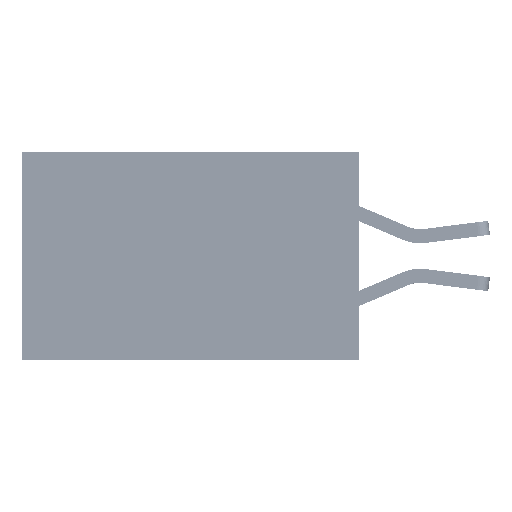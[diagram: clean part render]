
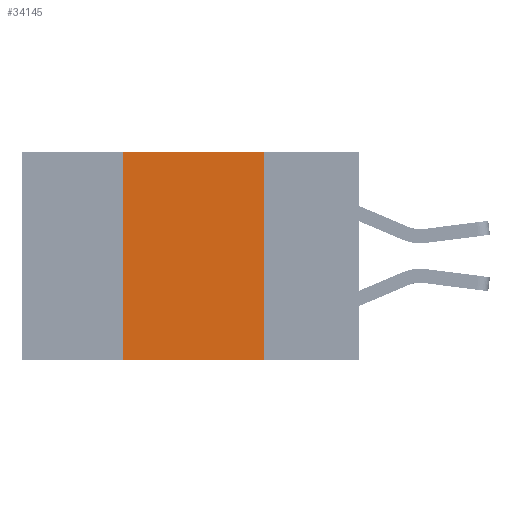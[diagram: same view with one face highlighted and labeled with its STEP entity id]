
A CAD part, left-side view. The second image highlights one B-rep face of the part: STEP entity #34145.
In plain terms, the highlighted planar face has unit normal (-1, 0, 0).
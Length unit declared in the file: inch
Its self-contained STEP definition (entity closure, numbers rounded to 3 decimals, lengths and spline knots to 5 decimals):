
#347 = VECTOR ( 'NONE', #7726, 39.37008 ) ;
#1479 = EDGE_CURVE ( 'NONE', #6688, #5592, #26765, .T. ) ;
#2944 = ORIENTED_EDGE ( 'NONE', *, *, #46217, .F. ) ;
#4751 = ORIENTED_EDGE ( 'NONE', *, *, #13920, .T. ) ;
#5285 = LINE ( 'NONE', #10228, #30888 ) ;
#5592 = VERTEX_POINT ( 'NONE', #26755 ) ;
#6181 = DIRECTION ( 'NONE',  ( 0., -1., 0. ) ) ;
#6688 = VERTEX_POINT ( 'NONE', #30655 ) ;
#7215 = DIRECTION ( 'NONE',  ( 1., 0., 0. ) ) ;
#7460 = PLANE ( 'NONE',  #26690 ) ;
#7726 = DIRECTION ( 'NONE',  ( 0., -1., 0. ) ) ;
#7950 = FACE_OUTER_BOUND ( 'NONE', #32301, .T. ) ;
#8558 = DIRECTION ( 'NONE',  ( 0., 0., 1. ) ) ;
#10228 = CARTESIAN_POINT ( 'NONE',  ( 0., 0.42, 0. ) ) ;
#10901 = DIRECTION ( 'NONE',  ( 0., 0., -1. ) ) ;
#13920 = EDGE_CURVE ( 'NONE', #14636, #22866, #25231, .T. ) ;
#14636 = VERTEX_POINT ( 'NONE', #47367 ) ;
#22866 = VERTEX_POINT ( 'NONE', #38891 ) ;
#24847 = VECTOR ( 'NONE', #6181, 39.37008 ) ;
#25231 = LINE ( 'NONE', #40516, #24847 ) ;
#26690 = AXIS2_PLACEMENT_3D ( 'NONE', #45314, #7215, #37519 ) ;
#26755 = CARTESIAN_POINT ( 'NONE',  ( 0., 0.17, 0. ) ) ;
#26765 = LINE ( 'NONE', #42049, #347 ) ;
#29707 = LINE ( 'NONE', #32953, #30104 ) ;
#30104 = VECTOR ( 'NONE', #10901, 39.37008 ) ;
#30655 = CARTESIAN_POINT ( 'NONE',  ( 0., 0.42, 0. ) ) ;
#30888 = VECTOR ( 'NONE', #8558, 39.37008 ) ;
#32301 = EDGE_LOOP ( 'NONE', ( #33962, #37680, #2944, #4751 ) ) ;
#32953 = CARTESIAN_POINT ( 'NONE',  ( 0., 0.17, 0. ) ) ;
#33962 = ORIENTED_EDGE ( 'NONE', *, *, #48400, .F. ) ;
#34145 = ADVANCED_FACE ( 'NONE', ( #7950 ), #7460, .F. ) ;
#37519 = DIRECTION ( 'NONE',  ( 0., 0., -1. ) ) ;
#37680 = ORIENTED_EDGE ( 'NONE', *, *, #1479, .F. ) ;
#38891 = CARTESIAN_POINT ( 'NONE',  ( 0., 0.17, -0.37 ) ) ;
#40516 = CARTESIAN_POINT ( 'NONE',  ( 0., 0.6, -0.37 ) ) ;
#42049 = CARTESIAN_POINT ( 'NONE',  ( 0., 0.6, 0. ) ) ;
#45314 = CARTESIAN_POINT ( 'NONE',  ( 0., 0.6, 0. ) ) ;
#46217 = EDGE_CURVE ( 'NONE', #14636, #6688, #5285, .T. ) ;
#47367 = CARTESIAN_POINT ( 'NONE',  ( 0., 0.42, -0.37 ) ) ;
#48400 = EDGE_CURVE ( 'NONE', #5592, #22866, #29707, .T. ) ;
